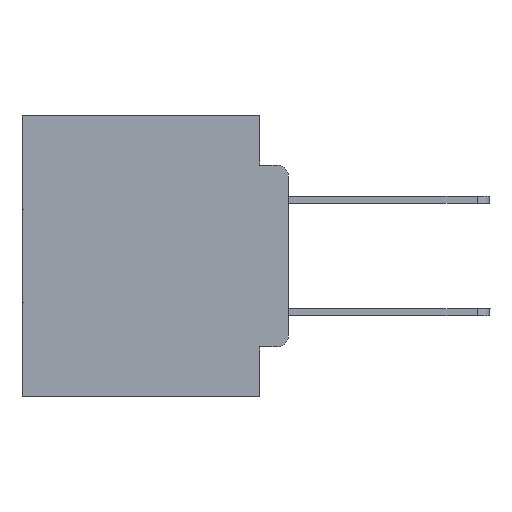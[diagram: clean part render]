
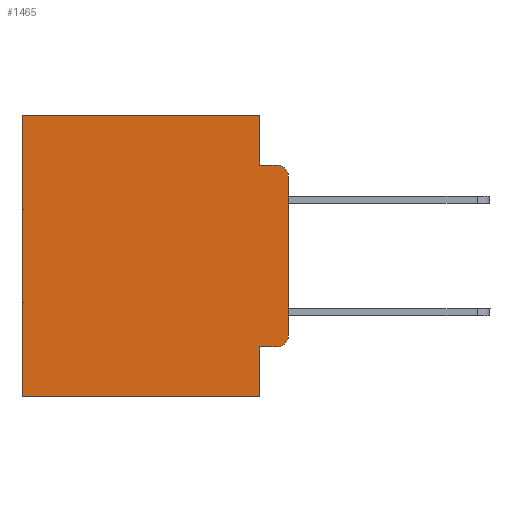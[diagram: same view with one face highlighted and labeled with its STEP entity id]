
A CAD part, left-side view. The second image highlights one B-rep face of the part: STEP entity #1465.
In plain terms, the highlighted planar face has unit normal (-1, 0, 0).
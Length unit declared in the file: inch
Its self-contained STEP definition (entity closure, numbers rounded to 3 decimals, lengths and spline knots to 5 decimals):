
#642 = CARTESIAN_POINT ( 'NONE',  ( 0.298, 0.051, -0.5 ) ) ;
#1279 = DIRECTION ( 'NONE',  ( 0., 0., -1. ) ) ;
#1338 = PLANE ( 'NONE',  #2030 ) ;
#1465 = ADVANCED_FACE ( 'NONE', ( #15737 ), #1338, .F. ) ;
#2030 = AXIS2_PLACEMENT_3D ( 'NONE', #20634, #8479, #13465 ) ;
#3118 = VERTEX_POINT ( 'NONE', #20944 ) ;
#4332 = VECTOR ( 'NONE', #18583, 39.37008 ) ;
#4826 = DIRECTION ( 'NONE',  ( 0., 0., -1. ) ) ;
#4886 = EDGE_CURVE ( 'NONE', #24497, #13914, #15473, .T. ) ;
#4956 = VERTEX_POINT ( 'NONE', #18522 ) ;
#4993 = DIRECTION ( 'NONE',  ( 0., 0., -1. ) ) ;
#5315 = LINE ( 'NONE', #27306, #9796 ) ;
#5423 = CARTESIAN_POINT ( 'NONE',  ( 0.298, 0., 0. ) ) ;
#5681 = ORIENTED_EDGE ( 'NONE', *, *, #25411, .F. ) ;
#6132 = ORIENTED_EDGE ( 'NONE', *, *, #15985, .F. ) ;
#6236 = VECTOR ( 'NONE', #27035, 39.37008 ) ;
#6884 = VECTOR ( 'NONE', #1279, 39.37008 ) ;
#7342 = DIRECTION ( 'NONE',  ( -1., 0., 0. ) ) ;
#8007 = CARTESIAN_POINT ( 'NONE',  ( 0.298, 0.473, 0. ) ) ;
#8250 = VERTEX_POINT ( 'NONE', #642 ) ;
#8479 = DIRECTION ( 'NONE',  ( 1., 0., 0. ) ) ;
#8938 = CARTESIAN_POINT ( 'NONE',  ( 0.298, 0.051, -0.0885 ) ) ;
#9134 = VECTOR ( 'NONE', #11448, 39.37008 ) ;
#9796 = VECTOR ( 'NONE', #12583, 39.37008 ) ;
#9816 = ORIENTED_EDGE ( 'NONE', *, *, #12832, .T. ) ;
#10673 = CARTESIAN_POINT ( 'NONE',  ( 0.298, 0.051, 0. ) ) ;
#10945 = CARTESIAN_POINT ( 'NONE',  ( 0.298, 0.051, -0.4115 ) ) ;
#11009 = EDGE_CURVE ( 'NONE', #4956, #22201, #29131, .T. ) ;
#11410 = CARTESIAN_POINT ( 'NONE',  ( 0.298, 0.051, -0.4115 ) ) ;
#11448 = DIRECTION ( 'NONE',  ( 0., -1., 0. ) ) ;
#11676 = ORIENTED_EDGE ( 'NONE', *, *, #22239, .T. ) ;
#12058 = DIRECTION ( 'NONE',  ( 0., 0., -1. ) ) ;
#12129 = LINE ( 'NONE', #15785, #6884 ) ;
#12278 = CARTESIAN_POINT ( 'NONE',  ( 0.298, 0.051, -0.0885 ) ) ;
#12548 = EDGE_LOOP ( 'NONE', ( #28464, #11676, #17050, #19398, #28551, #14586, #6132, #5681, #9816, #28687 ) ) ;
#12583 = DIRECTION ( 'NONE',  ( 0., 1., 0. ) ) ;
#12624 = LINE ( 'NONE', #28754, #20803 ) ;
#12832 = EDGE_CURVE ( 'NONE', #18854, #4956, #29773, .T. ) ;
#13130 = EDGE_CURVE ( 'NONE', #17687, #18496, #15157, .T. ) ;
#13465 = DIRECTION ( 'NONE',  ( 0., 0., -1. ) ) ;
#13576 = CARTESIAN_POINT ( 'NONE',  ( 0.298, 0.473, -0.5 ) ) ;
#13914 = VERTEX_POINT ( 'NONE', #22823 ) ;
#14324 = CARTESIAN_POINT ( 'NONE',  ( 0.298, 0., -0.3915 ) ) ;
#14502 = CARTESIAN_POINT ( 'NONE',  ( 0.298, 0.02, -0.3915 ) ) ;
#14586 = ORIENTED_EDGE ( 'NONE', *, *, #19177, .T. ) ;
#15157 = LINE ( 'NONE', #5423, #6236 ) ;
#15473 = LINE ( 'NONE', #8938, #9134 ) ;
#15737 = FACE_OUTER_BOUND ( 'NONE', #12548, .T. ) ;
#15785 = CARTESIAN_POINT ( 'NONE',  ( 0.298, 0., 0. ) ) ;
#15985 = EDGE_CURVE ( 'NONE', #8250, #16972, #5315, .T. ) ;
#16307 = CARTESIAN_POINT ( 'NONE',  ( 0.298, 0.051, 0. ) ) ;
#16972 = VERTEX_POINT ( 'NONE', #13576 ) ;
#17050 = ORIENTED_EDGE ( 'NONE', *, *, #4886, .F. ) ;
#17105 = DIRECTION ( 'NONE',  ( -1., 0., 0. ) ) ;
#17687 = VERTEX_POINT ( 'NONE', #30551 ) ;
#18496 = VERTEX_POINT ( 'NONE', #8007 ) ;
#18522 = CARTESIAN_POINT ( 'NONE',  ( 0.298, 0.02, -0.4115 ) ) ;
#18583 = DIRECTION ( 'NONE',  ( 0., -1., 0. ) ) ;
#18854 = VERTEX_POINT ( 'NONE', #10945 ) ;
#19177 = EDGE_CURVE ( 'NONE', #18496, #16972, #12624, .T. ) ;
#19398 = ORIENTED_EDGE ( 'NONE', *, *, #28997, .F. ) ;
#19404 = CARTESIAN_POINT ( 'NONE',  ( 0.298, 0.02, -0.1085 ) ) ;
#19803 = LINE ( 'NONE', #16307, #28799 ) ;
#19873 = CIRCLE ( 'NONE', #23990, 0.02 ) ;
#20634 = CARTESIAN_POINT ( 'NONE',  ( 0.298, 0., 0. ) ) ;
#20803 = VECTOR ( 'NONE', #4826, 39.37008 ) ;
#20944 = CARTESIAN_POINT ( 'NONE',  ( 0.298, 0., -0.1085 ) ) ;
#22201 = VERTEX_POINT ( 'NONE', #14324 ) ;
#22239 = EDGE_CURVE ( 'NONE', #3118, #13914, #19873, .T. ) ;
#22823 = CARTESIAN_POINT ( 'NONE',  ( 0.298, 0.02, -0.0885 ) ) ;
#23523 = DIRECTION ( 'NONE',  ( 0., 0., -1. ) ) ;
#23990 = AXIS2_PLACEMENT_3D ( 'NONE', #19404, #7342, #12058 ) ;
#24138 = LINE ( 'NONE', #10673, #27518 ) ;
#24497 = VERTEX_POINT ( 'NONE', #12278 ) ;
#25411 = EDGE_CURVE ( 'NONE', #18854, #8250, #24138, .T. ) ;
#25723 = AXIS2_PLACEMENT_3D ( 'NONE', #14502, #17105, #4993 ) ;
#26634 = EDGE_CURVE ( 'NONE', #3118, #22201, #12129, .T. ) ;
#27035 = DIRECTION ( 'NONE',  ( 0., 1., 0. ) ) ;
#27306 = CARTESIAN_POINT ( 'NONE',  ( 0.298, 0., -0.5 ) ) ;
#27518 = VECTOR ( 'NONE', #29971, 39.37008 ) ;
#28464 = ORIENTED_EDGE ( 'NONE', *, *, #26634, .F. ) ;
#28551 = ORIENTED_EDGE ( 'NONE', *, *, #13130, .T. ) ;
#28687 = ORIENTED_EDGE ( 'NONE', *, *, #11009, .T. ) ;
#28754 = CARTESIAN_POINT ( 'NONE',  ( 0.298, 0.473, 0. ) ) ;
#28799 = VECTOR ( 'NONE', #23523, 39.37008 ) ;
#28997 = EDGE_CURVE ( 'NONE', #17687, #24497, #19803, .T. ) ;
#29131 = CIRCLE ( 'NONE', #25723, 0.02 ) ;
#29773 = LINE ( 'NONE', #11410, #4332 ) ;
#29971 = DIRECTION ( 'NONE',  ( 0., 0., -1. ) ) ;
#30551 = CARTESIAN_POINT ( 'NONE',  ( 0.298, 0.051, 0. ) ) ;
